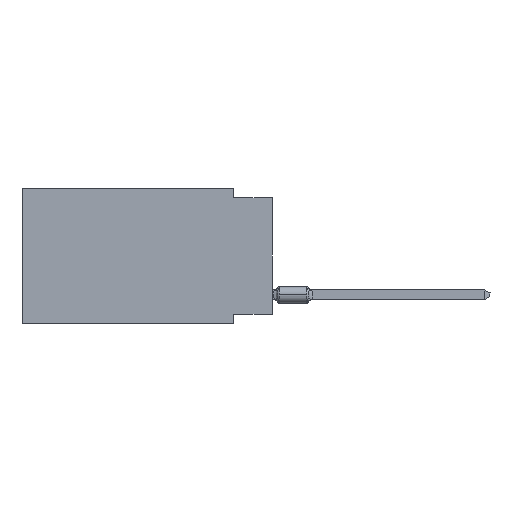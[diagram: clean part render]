
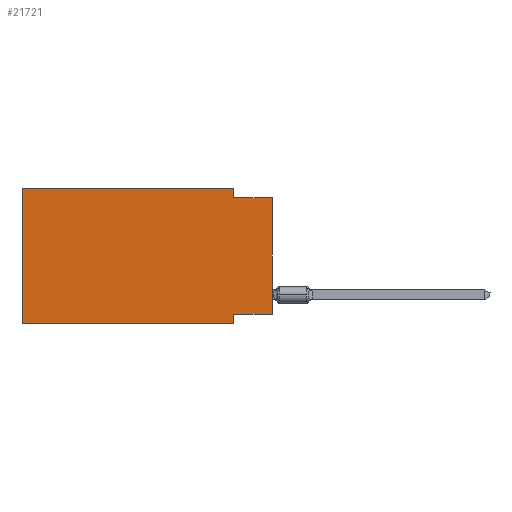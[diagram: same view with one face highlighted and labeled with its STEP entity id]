
A CAD part, left-side view. The second image highlights one B-rep face of the part: STEP entity #21721.
In plain terms, the highlighted planar face has unit normal (-1, 0, 0).
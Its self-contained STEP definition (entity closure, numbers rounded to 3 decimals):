
#707 = ORIENTED_EDGE ( 'NONE', *, *, #65773, .F. ) ;
#1875 = VECTOR ( 'NONE', #43059, 1000. ) ;
#2752 = LINE ( 'NONE', #19215, #48369 ) ;
#3665 = DIRECTION ( 'NONE',  ( 1., 0., 0. ) ) ;
#4366 = VECTOR ( 'NONE', #46551, 1000. ) ;
#5082 = CARTESIAN_POINT ( 'NONE',  ( 0., 2.54, -8.255 ) ) ;
#5660 = VERTEX_POINT ( 'NONE', #29486 ) ;
#7687 = CARTESIAN_POINT ( 'NONE',  ( 0., 2.54, 0. ) ) ;
#8787 = CARTESIAN_POINT ( 'NONE',  ( 0., 16.383, 0. ) ) ;
#9706 = VECTOR ( 'NONE', #27210, 1000. ) ;
#9841 = VECTOR ( 'NONE', #42578, 1000. ) ;
#9913 = VERTEX_POINT ( 'NONE', #58768 ) ;
#12213 = VERTEX_POINT ( 'NONE', #14949 ) ;
#14408 = DIRECTION ( 'NONE',  ( 0., 0., -1. ) ) ;
#14949 = CARTESIAN_POINT ( 'NONE',  ( 0., 16.383, -8.89 ) ) ;
#15013 = DIRECTION ( 'NONE',  ( 0., 0., 1. ) ) ;
#17860 = DIRECTION ( 'NONE',  ( 0., 0., 1. ) ) ;
#19215 = CARTESIAN_POINT ( 'NONE',  ( 0., 0., 0. ) ) ;
#19502 = EDGE_CURVE ( 'NONE', #12213, #35184, #43186, .T. ) ;
#20018 = LINE ( 'NONE', #26921, #1875 ) ;
#21721 = ADVANCED_FACE ( 'NONE', ( #43516 ), #42087, .F. ) ;
#22758 = ORIENTED_EDGE ( 'NONE', *, *, #47685, .F. ) ;
#23452 = CARTESIAN_POINT ( 'NONE',  ( 0., 0., -8.255 ) ) ;
#25019 = CARTESIAN_POINT ( 'NONE',  ( 0., 2.54, 0. ) ) ;
#25293 = VERTEX_POINT ( 'NONE', #7687 ) ;
#26187 = VERTEX_POINT ( 'NONE', #65926 ) ;
#26921 = CARTESIAN_POINT ( 'NONE',  ( 0., 2.54, -8.89 ) ) ;
#27048 = CARTESIAN_POINT ( 'NONE',  ( 0., 16.383, 0. ) ) ;
#27210 = DIRECTION ( 'NONE',  ( 0., -1., 0. ) ) ;
#27566 = LINE ( 'NONE', #33056, #9706 ) ;
#27806 = ORIENTED_EDGE ( 'NONE', *, *, #56412, .T. ) ;
#28883 = EDGE_LOOP ( 'NONE', ( #27806, #37629, #707, #46062, #37185, #66070, #22758, #53571 ) ) ;
#29243 = VERTEX_POINT ( 'NONE', #40496 ) ;
#29486 = CARTESIAN_POINT ( 'NONE',  ( 0., 2.54, -0.635 ) ) ;
#29962 = EDGE_CURVE ( 'NONE', #35184, #25293, #48789, .T. ) ;
#30385 = LINE ( 'NONE', #23452, #52829 ) ;
#33056 = CARTESIAN_POINT ( 'NONE',  ( 0., 16.383, -8.89 ) ) ;
#34815 = AXIS2_PLACEMENT_3D ( 'NONE', #8787, #3665, #70266 ) ;
#34892 = CARTESIAN_POINT ( 'NONE',  ( 0., 16.383, 0. ) ) ;
#35184 = VERTEX_POINT ( 'NONE', #34892 ) ;
#35516 = DIRECTION ( 'NONE',  ( 0., 1., 0. ) ) ;
#36302 = LINE ( 'NONE', #64121, #4366 ) ;
#37185 = ORIENTED_EDGE ( 'NONE', *, *, #19502, .F. ) ;
#37629 = ORIENTED_EDGE ( 'NONE', *, *, #37706, .F. ) ;
#37706 = EDGE_CURVE ( 'NONE', #5660, #26187, #36302, .T. ) ;
#39327 = VECTOR ( 'NONE', #15013, 1000. ) ;
#39612 = VERTEX_POINT ( 'NONE', #5082 ) ;
#40496 = CARTESIAN_POINT ( 'NONE',  ( 0., 0., -8.255 ) ) ;
#42087 = PLANE ( 'NONE',  #34815 ) ;
#42578 = DIRECTION ( 'NONE',  ( 0., -1., 0. ) ) ;
#43059 = DIRECTION ( 'NONE',  ( 0., 0., -1. ) ) ;
#43186 = LINE ( 'NONE', #27048, #39327 ) ;
#43516 = FACE_OUTER_BOUND ( 'NONE', #28883, .T. ) ;
#46062 = ORIENTED_EDGE ( 'NONE', *, *, #29962, .F. ) ;
#46551 = DIRECTION ( 'NONE',  ( 0., -1., 0. ) ) ;
#47685 = EDGE_CURVE ( 'NONE', #39612, #9913, #20018, .T. ) ;
#48369 = VECTOR ( 'NONE', #17860, 1000. ) ;
#48670 = VECTOR ( 'NONE', #14408, 1000. ) ;
#48789 = LINE ( 'NONE', #70404, #9841 ) ;
#52485 = LINE ( 'NONE', #25019, #48670 ) ;
#52829 = VECTOR ( 'NONE', #35516, 1000. ) ;
#53571 = ORIENTED_EDGE ( 'NONE', *, *, #54597, .F. ) ;
#54597 = EDGE_CURVE ( 'NONE', #29243, #39612, #30385, .T. ) ;
#56412 = EDGE_CURVE ( 'NONE', #29243, #26187, #2752, .T. ) ;
#58768 = CARTESIAN_POINT ( 'NONE',  ( 0., 2.54, -8.89 ) ) ;
#64121 = CARTESIAN_POINT ( 'NONE',  ( 0., 0., -0.635 ) ) ;
#65773 = EDGE_CURVE ( 'NONE', #25293, #5660, #52485, .T. ) ;
#65926 = CARTESIAN_POINT ( 'NONE',  ( 0., 0., -0.635 ) ) ;
#66070 = ORIENTED_EDGE ( 'NONE', *, *, #69654, .T. ) ;
#69654 = EDGE_CURVE ( 'NONE', #12213, #9913, #27566, .T. ) ;
#70266 = DIRECTION ( 'NONE',  ( 0., 0., -1. ) ) ;
#70404 = CARTESIAN_POINT ( 'NONE',  ( 0., 16.383, 0. ) ) ;
